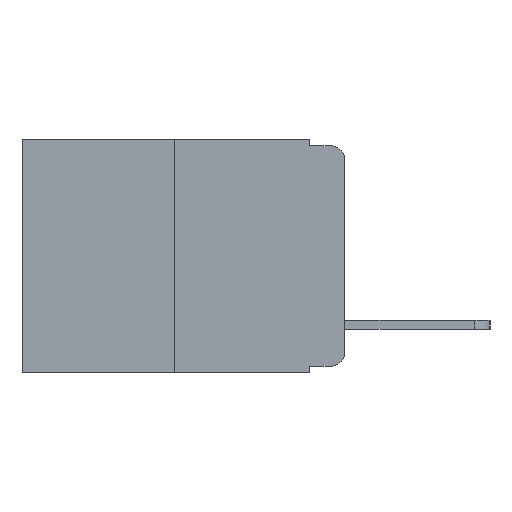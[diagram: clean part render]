
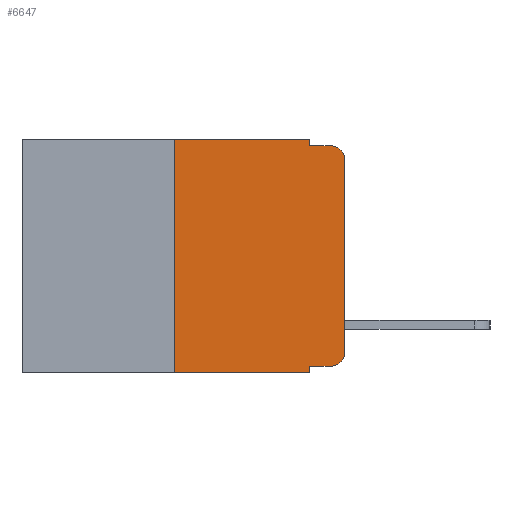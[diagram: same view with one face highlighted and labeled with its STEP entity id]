
A CAD part, left-side view. The second image highlights one B-rep face of the part: STEP entity #6647.
In plain terms, the highlighted planar face has unit normal (-1, 0, 0).
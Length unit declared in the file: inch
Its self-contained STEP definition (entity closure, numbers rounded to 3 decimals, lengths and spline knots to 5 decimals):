
#352 = DIRECTION ( 'NONE',  ( 0., 0., -1. ) ) ;
#369 = DIRECTION ( 'NONE',  ( -1., 0., 0. ) ) ;
#371 = CARTESIAN_POINT ( 'NONE',  ( 0., 0.02, -0.313 ) ) ;
#700 = ORIENTED_EDGE ( 'NONE', *, *, #9507, .F. ) ;
#935 = ORIENTED_EDGE ( 'NONE', *, *, #11167, .T. ) ;
#1019 = VERTEX_POINT ( 'NONE', #10499 ) ;
#1496 = ORIENTED_EDGE ( 'NONE', *, *, #8416, .F. ) ;
#1517 = VERTEX_POINT ( 'NONE', #7720 ) ;
#1612 = VERTEX_POINT ( 'NONE', #4063 ) ;
#1951 = VECTOR ( 'NONE', #9706, 39.37008 ) ;
#2106 = CARTESIAN_POINT ( 'NONE',  ( 0., 0.25, 0. ) ) ;
#2195 = CARTESIAN_POINT ( 'NONE',  ( 0., 0.02, -0.01 ) ) ;
#2288 = LINE ( 'NONE', #9754, #1951 ) ;
#2369 = ORIENTED_EDGE ( 'NONE', *, *, #11860, .T. ) ;
#2488 = AXIS2_PLACEMENT_3D ( 'NONE', #10542, #10310, #10279 ) ;
#2649 = VECTOR ( 'NONE', #11773, 39.37008 ) ;
#2658 = VERTEX_POINT ( 'NONE', #10997 ) ;
#2790 = ORIENTED_EDGE ( 'NONE', *, *, #9491, .F. ) ;
#2987 = ORIENTED_EDGE ( 'NONE', *, *, #9301, .T. ) ;
#3021 = ORIENTED_EDGE ( 'NONE', *, *, #9389, .T. ) ;
#3206 = LINE ( 'NONE', #11010, #8086 ) ;
#3309 = VERTEX_POINT ( 'NONE', #10121 ) ;
#3871 = VERTEX_POINT ( 'NONE', #2195 ) ;
#3902 = VECTOR ( 'NONE', #11035, 39.37008 ) ;
#4063 = CARTESIAN_POINT ( 'NONE',  ( 0., 0.051, 0. ) ) ;
#4071 = CARTESIAN_POINT ( 'NONE',  ( 0., 0.051, -0.01 ) ) ;
#4626 = VERTEX_POINT ( 'NONE', #2106 ) ;
#4849 = LINE ( 'NONE', #11548, #11498 ) ;
#5026 = EDGE_LOOP ( 'NONE', ( #2369, #5246, #6086, #6238, #1496, #700, #2987, #2790, #3021, #935 ) ) ;
#5246 = ORIENTED_EDGE ( 'NONE', *, *, #11762, .T. ) ;
#6086 = ORIENTED_EDGE ( 'NONE', *, *, #11743, .F. ) ;
#6204 = LINE ( 'NONE', #11047, #3902 ) ;
#6238 = ORIENTED_EDGE ( 'NONE', *, *, #9523, .F. ) ;
#6647 = ADVANCED_FACE ( 'NONE', ( #6950 ), #10246, .F. ) ;
#6950 = FACE_OUTER_BOUND ( 'NONE', #5026, .T. ) ;
#7521 = AXIS2_PLACEMENT_3D ( 'NONE', #10049, #10038, #10008 ) ;
#7720 = CARTESIAN_POINT ( 'NONE',  ( 0., 0., -0.313 ) ) ;
#7727 = CARTESIAN_POINT ( 'NONE',  ( 0., 0.02, -0.333 ) ) ;
#7814 = CARTESIAN_POINT ( 'NONE',  ( 0., 0., -0.03 ) ) ;
#7942 = VECTOR ( 'NONE', #10199, 39.37008 ) ;
#8086 = VECTOR ( 'NONE', #10968, 39.37008 ) ;
#8120 = VECTOR ( 'NONE', #8390, 39.37008 ) ;
#8161 = VERTEX_POINT ( 'NONE', #7814 ) ;
#8205 = LINE ( 'NONE', #10553, #7942 ) ;
#8355 = AXIS2_PLACEMENT_3D ( 'NONE', #371, #369, #352 ) ;
#8390 = DIRECTION ( 'NONE',  ( 0., -1., 0. ) ) ;
#8416 = EDGE_CURVE ( 'NONE', #4626, #1612, #10110, .T. ) ;
#8540 = CARTESIAN_POINT ( 'NONE',  ( 0., 0.473, 0. ) ) ;
#8618 = LINE ( 'NONE', #11137, #11004 ) ;
#9301 = EDGE_CURVE ( 'NONE', #1019, #2658, #10437, .T. ) ;
#9389 = EDGE_CURVE ( 'NONE', #3309, #9755, #4849, .T. ) ;
#9491 = EDGE_CURVE ( 'NONE', #3309, #2658, #8618, .T. ) ;
#9507 = EDGE_CURVE ( 'NONE', #1019, #4626, #6204, .T. ) ;
#9523 = EDGE_CURVE ( 'NONE', #1612, #10473, #3206, .T. ) ;
#9706 = DIRECTION ( 'NONE',  ( 0., 0., 1. ) ) ;
#9754 = CARTESIAN_POINT ( 'NONE',  ( 0., 0., 0. ) ) ;
#9755 = VERTEX_POINT ( 'NONE', #7727 ) ;
#10008 = DIRECTION ( 'NONE',  ( 0., 0., -1. ) ) ;
#10038 = DIRECTION ( 'NONE',  ( -1., 0., 0. ) ) ;
#10049 = CARTESIAN_POINT ( 'NONE',  ( 0., 0.02, -0.03 ) ) ;
#10110 = LINE ( 'NONE', #8540, #8120 ) ;
#10121 = CARTESIAN_POINT ( 'NONE',  ( 0., 0.051, -0.333 ) ) ;
#10181 = CIRCLE ( 'NONE', #7521, 0.02 ) ;
#10199 = DIRECTION ( 'NONE',  ( 0., -1., 0. ) ) ;
#10246 = PLANE ( 'NONE',  #2488 ) ;
#10279 = DIRECTION ( 'NONE',  ( 0., 0., -1. ) ) ;
#10310 = DIRECTION ( 'NONE',  ( 1., 0., 0. ) ) ;
#10437 = LINE ( 'NONE', #11969, #2649 ) ;
#10473 = VERTEX_POINT ( 'NONE', #4071 ) ;
#10499 = CARTESIAN_POINT ( 'NONE',  ( 0., 0.25, -0.343 ) ) ;
#10542 = CARTESIAN_POINT ( 'NONE',  ( 0., 0.473, 0. ) ) ;
#10553 = CARTESIAN_POINT ( 'NONE',  ( 0., 0.051, -0.01 ) ) ;
#10968 = DIRECTION ( 'NONE',  ( 0., 0., -1. ) ) ;
#10972 = CIRCLE ( 'NONE', #8355, 0.02 ) ;
#10997 = CARTESIAN_POINT ( 'NONE',  ( 0., 0.051, -0.343 ) ) ;
#11004 = VECTOR ( 'NONE', #11116, 39.37008 ) ;
#11010 = CARTESIAN_POINT ( 'NONE',  ( 0., 0.051, 0. ) ) ;
#11035 = DIRECTION ( 'NONE',  ( 0., 0., 1. ) ) ;
#11047 = CARTESIAN_POINT ( 'NONE',  ( 0., 0.25, 0. ) ) ;
#11116 = DIRECTION ( 'NONE',  ( 0., 0., -1. ) ) ;
#11137 = CARTESIAN_POINT ( 'NONE',  ( 0., 0.051, 0. ) ) ;
#11167 = EDGE_CURVE ( 'NONE', #9755, #1517, #10972, .T. ) ;
#11498 = VECTOR ( 'NONE', #11562, 39.37008 ) ;
#11548 = CARTESIAN_POINT ( 'NONE',  ( 0., 0.051, -0.333 ) ) ;
#11562 = DIRECTION ( 'NONE',  ( 0., -1., 0. ) ) ;
#11743 = EDGE_CURVE ( 'NONE', #10473, #3871, #8205, .T. ) ;
#11762 = EDGE_CURVE ( 'NONE', #8161, #3871, #10181, .T. ) ;
#11773 = DIRECTION ( 'NONE',  ( 0., -1., 0. ) ) ;
#11860 = EDGE_CURVE ( 'NONE', #1517, #8161, #2288, .T. ) ;
#11969 = CARTESIAN_POINT ( 'NONE',  ( 0., 0.473, -0.343 ) ) ;
